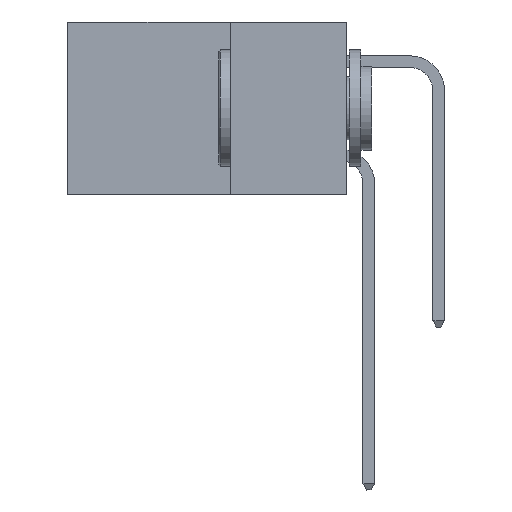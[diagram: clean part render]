
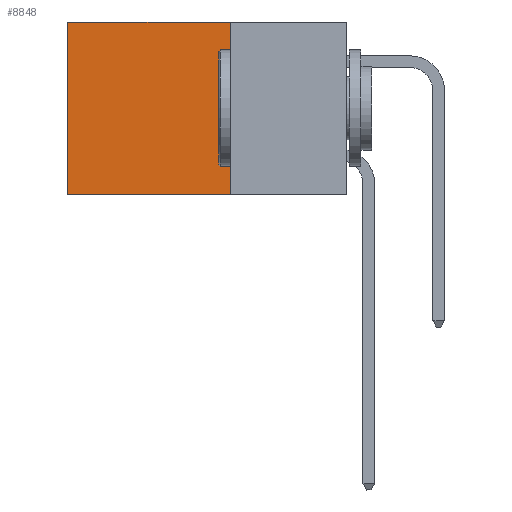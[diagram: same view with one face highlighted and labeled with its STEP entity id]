
A CAD part, left-side view. The second image highlights one B-rep face of the part: STEP entity #8848.
In plain terms, the highlighted planar face has unit normal (-1, 0, 0).
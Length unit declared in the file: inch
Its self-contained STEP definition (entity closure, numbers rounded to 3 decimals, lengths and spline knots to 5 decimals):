
#15 = DIRECTION ( 'NONE',  ( 0., 0., -1. ) ) ;
#95 = PLANE ( 'NONE',  #11197 ) ;
#757 = VERTEX_POINT ( 'NONE', #1259 ) ;
#998 = CARTESIAN_POINT ( 'NONE',  ( 0.2875, 0.25, -0.37 ) ) ;
#1259 = CARTESIAN_POINT ( 'NONE',  ( 0.2875, 0.6, -0.37 ) ) ;
#1703 = DIRECTION ( 'NONE',  ( 1., 0., 0. ) ) ;
#1711 = VECTOR ( 'NONE', #5549, 39.37008 ) ;
#1739 = LINE ( 'NONE', #1857, #4329 ) ;
#1857 = CARTESIAN_POINT ( 'NONE',  ( 0.2875, 0.25, 0. ) ) ;
#1875 = ORIENTED_EDGE ( 'NONE', *, *, #12902, .F. ) ;
#2235 = VERTEX_POINT ( 'NONE', #2918 ) ;
#2918 = CARTESIAN_POINT ( 'NONE',  ( 0.2875, 0.25, 0. ) ) ;
#2948 = CARTESIAN_POINT ( 'NONE',  ( 0.2875, 0.25, -0.37 ) ) ;
#3339 = CARTESIAN_POINT ( 'NONE',  ( 0.2875, 0.6, 0. ) ) ;
#3419 = VECTOR ( 'NONE', #12242, 39.37008 ) ;
#3585 = VERTEX_POINT ( 'NONE', #998 ) ;
#3796 = DIRECTION ( 'NONE',  ( 0., 0., -1. ) ) ;
#4329 = VECTOR ( 'NONE', #12036, 39.37008 ) ;
#5019 = VERTEX_POINT ( 'NONE', #3339 ) ;
#5549 = DIRECTION ( 'NONE',  ( 0., 1., 0. ) ) ;
#5699 = ORIENTED_EDGE ( 'NONE', *, *, #11953, .T. ) ;
#6019 = LINE ( 'NONE', #13329, #3419 ) ;
#7377 = ORIENTED_EDGE ( 'NONE', *, *, #14139, .T. ) ;
#7762 = LINE ( 'NONE', #2948, #1711 ) ;
#7845 = CARTESIAN_POINT ( 'NONE',  ( 0.2875, 0.25, 0. ) ) ;
#8848 = ADVANCED_FACE ( 'NONE', ( #9018 ), #95, .F. ) ;
#9018 = FACE_OUTER_BOUND ( 'NONE', #12106, .T. ) ;
#9024 = LINE ( 'NONE', #11211, #11520 ) ;
#11197 = AXIS2_PLACEMENT_3D ( 'NONE', #7845, #1703, #3796 ) ;
#11211 = CARTESIAN_POINT ( 'NONE',  ( 0.2875, 0.25, 0. ) ) ;
#11499 = EDGE_CURVE ( 'NONE', #2235, #3585, #9024, .T. ) ;
#11520 = VECTOR ( 'NONE', #15, 39.37008 ) ;
#11953 = EDGE_CURVE ( 'NONE', #2235, #5019, #1739, .T. ) ;
#12036 = DIRECTION ( 'NONE',  ( 0., 1., 0. ) ) ;
#12106 = EDGE_LOOP ( 'NONE', ( #7377, #1875, #12797, #5699 ) ) ;
#12242 = DIRECTION ( 'NONE',  ( 0., 0., -1. ) ) ;
#12797 = ORIENTED_EDGE ( 'NONE', *, *, #11499, .F. ) ;
#12902 = EDGE_CURVE ( 'NONE', #3585, #757, #7762, .T. ) ;
#13329 = CARTESIAN_POINT ( 'NONE',  ( 0.2875, 0.6, 0. ) ) ;
#14139 = EDGE_CURVE ( 'NONE', #5019, #757, #6019, .T. ) ;
